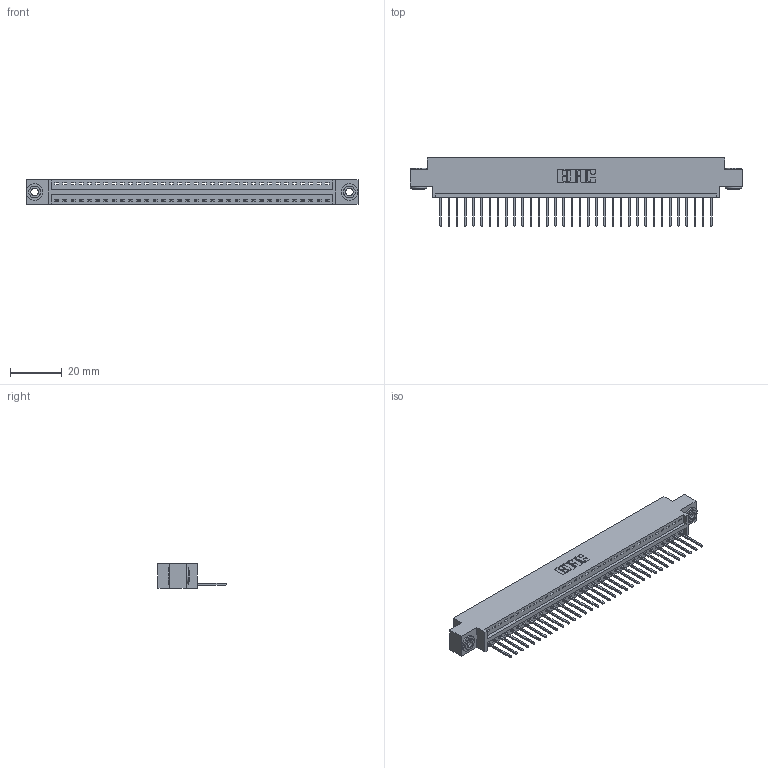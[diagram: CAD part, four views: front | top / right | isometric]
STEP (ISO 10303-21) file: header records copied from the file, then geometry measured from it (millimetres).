
FILE_DESCRIPTION (( 'STEP AP203' ), '1' );
FILE_NAME ('346-034-522-603.STEP', '2022-05-06T21:15:12', ( '' ), ( '' ), 'SwSTEP 2.0', 'SolidWorks 2020', '' );
FILE_SCHEMA (( 'CONFIG_CONTROL_DESIGN' ));
Length unit declared in the file: inch
Products named in the file (4): 345-250-002_345-250-002-102; 346 Part_0.170 Offset - 0.156 Dia-TH; 345-292-001_345-293-122; 346-034-522-603
Assembly tree (37 placements, depth 2):
  346-034-522-603
    346 Part_0.170 Offset - 0.156 Dia-TH
    345-292-001_345-293-122  x34
    345-250-002_345-250-002-102  x2
Bounding box: 128.52 x 26.42 x 9.4 mm (x, y, z)
Volume: 12098.4 mm3; surface area: 15572.1 mm2
Topology: 37 solids, 37 shells, 2150 faces, 6437 edges, 4242 vertices
Faces by surface type: plane 1464, cylinder 678, cone 8
Entity records: 23394 total; most frequent: CARTESIAN_POINT 3995, ORIENTED_EDGE 3954, DIRECTION 3563, EDGE_CURVE 1977, LINE 1685, VECTOR 1685, VERTEX_POINT 1314, AXIS2_PLACEMENT_3D 939
